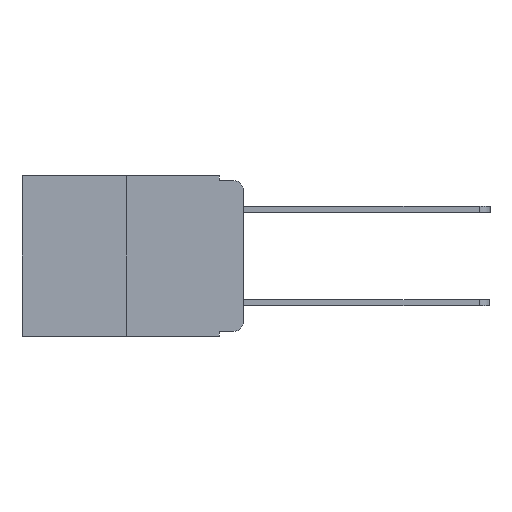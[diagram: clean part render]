
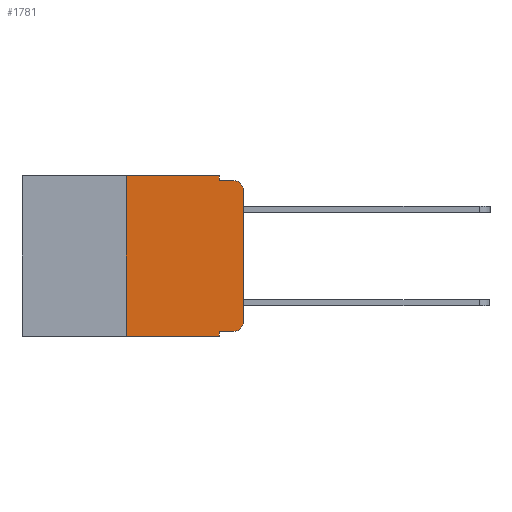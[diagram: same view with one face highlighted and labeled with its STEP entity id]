
A CAD part, left-side view. The second image highlights one B-rep face of the part: STEP entity #1781.
In plain terms, the highlighted planar face has unit normal (-1, 0, 0).
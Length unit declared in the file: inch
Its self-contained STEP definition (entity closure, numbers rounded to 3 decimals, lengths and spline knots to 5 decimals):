
#10 = ORIENTED_EDGE ( 'NONE', *, *, #1247, .T. ) ;
#303 = VECTOR ( 'NONE', #3850, 39.37008 ) ;
#348 = EDGE_CURVE ( 'NONE', #891, #7735, #5421, .T. ) ;
#667 = DIRECTION ( 'NONE',  ( 0., 0., -1. ) ) ;
#768 = CARTESIAN_POINT ( 'NONE',  ( 0., 0.051, -0.01 ) ) ;
#813 = CARTESIAN_POINT ( 'NONE',  ( 0., 0.25, 0. ) ) ;
#891 = VERTEX_POINT ( 'NONE', #9198 ) ;
#1247 = EDGE_CURVE ( 'NONE', #4631, #11883, #4332, .T. ) ;
#1268 = CARTESIAN_POINT ( 'NONE',  ( 0., 0.473, 0. ) ) ;
#1393 = DIRECTION ( 'NONE',  ( 0., 0., -1. ) ) ;
#1404 = EDGE_CURVE ( 'NONE', #11883, #7896, #4804, .T. ) ;
#1506 = ORIENTED_EDGE ( 'NONE', *, *, #348, .F. ) ;
#1552 = DIRECTION ( 'NONE',  ( 0., 0., -1. ) ) ;
#1570 = LINE ( 'NONE', #6855, #11297 ) ;
#1732 = ORIENTED_EDGE ( 'NONE', *, *, #5948, .F. ) ;
#1781 = ADVANCED_FACE ( 'NONE', ( #3071 ), #8193, .F. ) ;
#1851 = CARTESIAN_POINT ( 'NONE',  ( 0., 0., -0.313 ) ) ;
#2092 = AXIS2_PLACEMENT_3D ( 'NONE', #11991, #6571, #667 ) ;
#2420 = CARTESIAN_POINT ( 'NONE',  ( 0., 0.051, -0.333 ) ) ;
#2503 = ORIENTED_EDGE ( 'NONE', *, *, #10951, .F. ) ;
#2881 = EDGE_CURVE ( 'NONE', #4631, #9503, #9773, .T. ) ;
#3071 = FACE_OUTER_BOUND ( 'NONE', #8048, .T. ) ;
#3090 = VECTOR ( 'NONE', #1552, 39.37008 ) ;
#3338 = ORIENTED_EDGE ( 'NONE', *, *, #6335, .T. ) ;
#3434 = CARTESIAN_POINT ( 'NONE',  ( 0., 0.051, -0.333 ) ) ;
#3614 = DIRECTION ( 'NONE',  ( 0., -1., 0. ) ) ;
#3850 = DIRECTION ( 'NONE',  ( 0., 0., 1. ) ) ;
#3866 = ORIENTED_EDGE ( 'NONE', *, *, #2881, .F. ) ;
#3995 = LINE ( 'NONE', #8491, #303 ) ;
#4307 = DIRECTION ( 'NONE',  ( 0., -1., 0. ) ) ;
#4332 = LINE ( 'NONE', #2420, #11384 ) ;
#4361 = ORIENTED_EDGE ( 'NONE', *, *, #1404, .T. ) ;
#4397 = ORIENTED_EDGE ( 'NONE', *, *, #7049, .T. ) ;
#4432 = VERTEX_POINT ( 'NONE', #10579 ) ;
#4631 = VERTEX_POINT ( 'NONE', #3434 ) ;
#4804 = CIRCLE ( 'NONE', #8200, 0.02 ) ;
#5212 = VECTOR ( 'NONE', #4307, 39.37008 ) ;
#5264 = DIRECTION ( 'NONE',  ( 0., 0., 1. ) ) ;
#5421 = LINE ( 'NONE', #768, #7862 ) ;
#5686 = LINE ( 'NONE', #11839, #3090 ) ;
#5722 = CIRCLE ( 'NONE', #2092, 0.02 ) ;
#5948 = EDGE_CURVE ( 'NONE', #10955, #10669, #1570, .T. ) ;
#6335 = EDGE_CURVE ( 'NONE', #9478, #7735, #5722, .T. ) ;
#6571 = DIRECTION ( 'NONE',  ( -1., 0., 0. ) ) ;
#6611 = ORIENTED_EDGE ( 'NONE', *, *, #10640, .T. ) ;
#6855 = CARTESIAN_POINT ( 'NONE',  ( 0., 0.25, 0. ) ) ;
#6908 = CARTESIAN_POINT ( 'NONE',  ( 0., 0., -0.03 ) ) ;
#6995 = LINE ( 'NONE', #11045, #11011 ) ;
#7049 = EDGE_CURVE ( 'NONE', #10955, #9503, #6995, .T. ) ;
#7203 = DIRECTION ( 'NONE',  ( -1., 0., 0. ) ) ;
#7279 = CARTESIAN_POINT ( 'NONE',  ( 0., 0.02, -0.313 ) ) ;
#7330 = VECTOR ( 'NONE', #10257, 39.37008 ) ;
#7652 = LINE ( 'NONE', #1268, #5212 ) ;
#7735 = VERTEX_POINT ( 'NONE', #11929 ) ;
#7862 = VECTOR ( 'NONE', #10345, 39.37008 ) ;
#7896 = VERTEX_POINT ( 'NONE', #1851 ) ;
#8048 = EDGE_LOOP ( 'NONE', ( #6611, #3338, #1506, #10220, #2503, #1732, #4397, #3866, #10, #4361 ) ) ;
#8193 = PLANE ( 'NONE',  #10202 ) ;
#8200 = AXIS2_PLACEMENT_3D ( 'NONE', #7279, #7203, #1393 ) ;
#8412 = EDGE_CURVE ( 'NONE', #4432, #891, #5686, .T. ) ;
#8491 = CARTESIAN_POINT ( 'NONE',  ( 0., 0., 0. ) ) ;
#8635 = CARTESIAN_POINT ( 'NONE',  ( 0., 0.02, -0.333 ) ) ;
#9198 = CARTESIAN_POINT ( 'NONE',  ( 0., 0.051, -0.01 ) ) ;
#9333 = CARTESIAN_POINT ( 'NONE',  ( 0., 0.051, 0. ) ) ;
#9478 = VERTEX_POINT ( 'NONE', #6908 ) ;
#9503 = VERTEX_POINT ( 'NONE', #11483 ) ;
#9773 = LINE ( 'NONE', #9333, #7330 ) ;
#10135 = DIRECTION ( 'NONE',  ( 1., 0., 0. ) ) ;
#10202 = AXIS2_PLACEMENT_3D ( 'NONE', #10570, #10135, #12228 ) ;
#10220 = ORIENTED_EDGE ( 'NONE', *, *, #8412, .F. ) ;
#10257 = DIRECTION ( 'NONE',  ( 0., 0., -1. ) ) ;
#10345 = DIRECTION ( 'NONE',  ( 0., -1., 0. ) ) ;
#10570 = CARTESIAN_POINT ( 'NONE',  ( 0., 0.473, 0. ) ) ;
#10579 = CARTESIAN_POINT ( 'NONE',  ( 0., 0.051, 0. ) ) ;
#10640 = EDGE_CURVE ( 'NONE', #7896, #9478, #3995, .T. ) ;
#10669 = VERTEX_POINT ( 'NONE', #813 ) ;
#10951 = EDGE_CURVE ( 'NONE', #10669, #4432, #7652, .T. ) ;
#10955 = VERTEX_POINT ( 'NONE', #11602 ) ;
#11011 = VECTOR ( 'NONE', #3614, 39.37008 ) ;
#11045 = CARTESIAN_POINT ( 'NONE',  ( 0., 0.473, -0.343 ) ) ;
#11297 = VECTOR ( 'NONE', #5264, 39.37008 ) ;
#11384 = VECTOR ( 'NONE', #11659, 39.37008 ) ;
#11483 = CARTESIAN_POINT ( 'NONE',  ( 0., 0.051, -0.343 ) ) ;
#11602 = CARTESIAN_POINT ( 'NONE',  ( 0., 0.25, -0.343 ) ) ;
#11659 = DIRECTION ( 'NONE',  ( 0., -1., 0. ) ) ;
#11839 = CARTESIAN_POINT ( 'NONE',  ( 0., 0.051, 0. ) ) ;
#11883 = VERTEX_POINT ( 'NONE', #8635 ) ;
#11929 = CARTESIAN_POINT ( 'NONE',  ( 0., 0.02, -0.01 ) ) ;
#11991 = CARTESIAN_POINT ( 'NONE',  ( 0., 0.02, -0.03 ) ) ;
#12228 = DIRECTION ( 'NONE',  ( 0., 0., -1. ) ) ;
